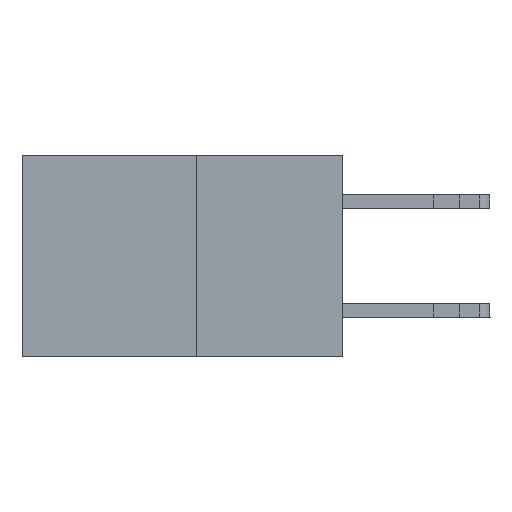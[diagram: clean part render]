
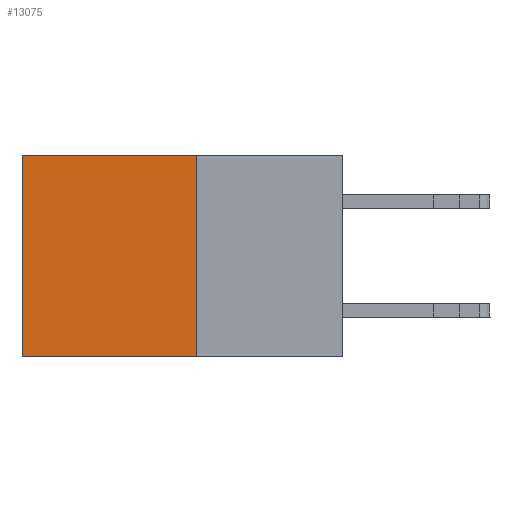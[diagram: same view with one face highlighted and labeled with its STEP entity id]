
A CAD part, left-side view. The second image highlights one B-rep face of the part: STEP entity #13075.
In plain terms, the highlighted planar face has unit normal (-1, 0, 0).
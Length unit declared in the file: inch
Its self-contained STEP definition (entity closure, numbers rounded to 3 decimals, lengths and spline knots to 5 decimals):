
#965 = EDGE_CURVE ( 'NONE', #9795, #15896, #16550, .T. ) ;
#2158 = CARTESIAN_POINT ( 'NONE',  ( 0.277, 0.59, 0. ) ) ;
#2356 = CARTESIAN_POINT ( 'NONE',  ( 0.277, 0.59, -0.37 ) ) ;
#2957 = ORIENTED_EDGE ( 'NONE', *, *, #14273, .T. ) ;
#2994 = VERTEX_POINT ( 'NONE', #2158 ) ;
#3140 = ORIENTED_EDGE ( 'NONE', *, *, #965, .F. ) ;
#3161 = LINE ( 'NONE', #18942, #7555 ) ;
#3410 = LINE ( 'NONE', #8882, #7230 ) ;
#4374 = FACE_OUTER_BOUND ( 'NONE', #18591, .T. ) ;
#4557 = VERTEX_POINT ( 'NONE', #23295 ) ;
#5203 = AXIS2_PLACEMENT_3D ( 'NONE', #16300, #16217, #16135 ) ;
#5386 = ORIENTED_EDGE ( 'NONE', *, *, #22332, .F. ) ;
#7230 = VECTOR ( 'NONE', #14492, 39.37008 ) ;
#7516 = VECTOR ( 'NONE', #20385, 39.37008 ) ;
#7555 = VECTOR ( 'NONE', #9599, 39.37008 ) ;
#8882 = CARTESIAN_POINT ( 'NONE',  ( 0.277, 0.27, 0. ) ) ;
#9599 = DIRECTION ( 'NONE',  ( 0., 0., -1. ) ) ;
#9795 = VERTEX_POINT ( 'NONE', #21991 ) ;
#11572 = VECTOR ( 'NONE', #17599, 39.37008 ) ;
#12049 = CARTESIAN_POINT ( 'NONE',  ( 0.277, 0.27, -0.37 ) ) ;
#12447 = LINE ( 'NONE', #14679, #7516 ) ;
#13075 = ADVANCED_FACE ( 'NONE', ( #4374 ), #16467, .F. ) ;
#14273 = EDGE_CURVE ( 'NONE', #4557, #2994, #3410, .T. ) ;
#14492 = DIRECTION ( 'NONE',  ( 0., 1., 0. ) ) ;
#14679 = CARTESIAN_POINT ( 'NONE',  ( 0.277, 0.59, -0.37 ) ) ;
#15896 = VERTEX_POINT ( 'NONE', #2356 ) ;
#16135 = DIRECTION ( 'NONE',  ( 0., 0., -1. ) ) ;
#16217 = DIRECTION ( 'NONE',  ( 1., 0., 0. ) ) ;
#16300 = CARTESIAN_POINT ( 'NONE',  ( 0.277, 0.27, -0.37 ) ) ;
#16467 = PLANE ( 'NONE',  #5203 ) ;
#16550 = LINE ( 'NONE', #12049, #11572 ) ;
#17599 = DIRECTION ( 'NONE',  ( 0., 1., 0. ) ) ;
#18591 = EDGE_LOOP ( 'NONE', ( #20247, #3140, #5386, #2957 ) ) ;
#18942 = CARTESIAN_POINT ( 'NONE',  ( 0.277, 0.27, -0.37 ) ) ;
#20247 = ORIENTED_EDGE ( 'NONE', *, *, #23205, .T. ) ;
#20385 = DIRECTION ( 'NONE',  ( 0., 0., -1. ) ) ;
#21991 = CARTESIAN_POINT ( 'NONE',  ( 0.277, 0.27, -0.37 ) ) ;
#22332 = EDGE_CURVE ( 'NONE', #4557, #9795, #3161, .T. ) ;
#23205 = EDGE_CURVE ( 'NONE', #2994, #15896, #12447, .T. ) ;
#23295 = CARTESIAN_POINT ( 'NONE',  ( 0.277, 0.27, 0. ) ) ;
